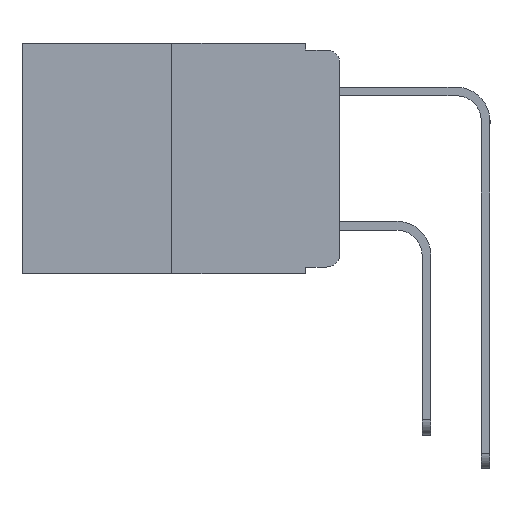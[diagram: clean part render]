
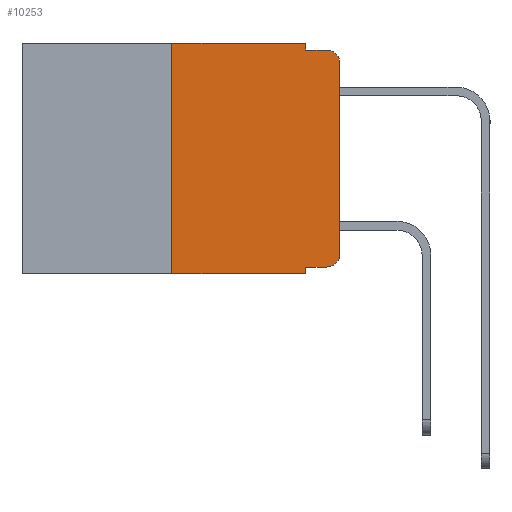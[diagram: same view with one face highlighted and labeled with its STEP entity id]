
A CAD part, left-side view. The second image highlights one B-rep face of the part: STEP entity #10253.
In plain terms, the highlighted planar face has unit normal (-1, 0, 0).
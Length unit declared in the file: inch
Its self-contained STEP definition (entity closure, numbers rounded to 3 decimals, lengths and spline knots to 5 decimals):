
#433 = CARTESIAN_POINT ( 'NONE',  ( 0., 0.02, -0.333 ) ) ;
#445 = VERTEX_POINT ( 'NONE', #18085 ) ;
#580 = VERTEX_POINT ( 'NONE', #11649 ) ;
#605 = CARTESIAN_POINT ( 'NONE',  ( 0., 0.051, -0.01 ) ) ;
#754 = ORIENTED_EDGE ( 'NONE', *, *, #6500, .T. ) ;
#1290 = CARTESIAN_POINT ( 'NONE',  ( 0., 0.051, 0. ) ) ;
#1315 = EDGE_CURVE ( 'NONE', #15771, #9281, #1794, .T. ) ;
#1666 = CARTESIAN_POINT ( 'NONE',  ( 0., 0.473, 0. ) ) ;
#1714 = CARTESIAN_POINT ( 'NONE',  ( 0., 0.02, -0.03 ) ) ;
#1794 = LINE ( 'NONE', #10385, #9416 ) ;
#2093 = VECTOR ( 'NONE', #3035, 39.37008 ) ;
#2310 = ORIENTED_EDGE ( 'NONE', *, *, #16106, .F. ) ;
#2393 = CARTESIAN_POINT ( 'NONE',  ( 0., 0., -0.03 ) ) ;
#2771 = LINE ( 'NONE', #4228, #17580 ) ;
#2991 = DIRECTION ( 'NONE',  ( -1., 0., 0. ) ) ;
#3035 = DIRECTION ( 'NONE',  ( 0., -1., 0. ) ) ;
#3064 = EDGE_CURVE ( 'NONE', #445, #11190, #14679, .T. ) ;
#3066 = ORIENTED_EDGE ( 'NONE', *, *, #5464, .T. ) ;
#3244 = DIRECTION ( 'NONE',  ( 1., 0., 0. ) ) ;
#3263 = CARTESIAN_POINT ( 'NONE',  ( 0., 0., 0. ) ) ;
#3291 = DIRECTION ( 'NONE',  ( 0., 0., -1. ) ) ;
#4115 = EDGE_CURVE ( 'NONE', #5108, #580, #12930, .T. ) ;
#4228 = CARTESIAN_POINT ( 'NONE',  ( 0., 0.25, 0. ) ) ;
#4247 = AXIS2_PLACEMENT_3D ( 'NONE', #1714, #12089, #3291 ) ;
#4293 = EDGE_CURVE ( 'NONE', #14950, #5108, #17659, .T. ) ;
#4576 = CARTESIAN_POINT ( 'NONE',  ( 0., 0.473, 0. ) ) ;
#4803 = DIRECTION ( 'NONE',  ( 0., 0., 1. ) ) ;
#4983 = DIRECTION ( 'NONE',  ( 0., -1., 0. ) ) ;
#5108 = VERTEX_POINT ( 'NONE', #433 ) ;
#5315 = EDGE_CURVE ( 'NONE', #14950, #11190, #12246, .T. ) ;
#5464 = EDGE_CURVE ( 'NONE', #6756, #9281, #12873, .T. ) ;
#5842 = VECTOR ( 'NONE', #6880, 39.37008 ) ;
#5884 = ORIENTED_EDGE ( 'NONE', *, *, #4293, .T. ) ;
#6154 = LINE ( 'NONE', #4576, #2093 ) ;
#6315 = LINE ( 'NONE', #8388, #5842 ) ;
#6500 = EDGE_CURVE ( 'NONE', #580, #6756, #9173, .T. ) ;
#6756 = VERTEX_POINT ( 'NONE', #2393 ) ;
#6880 = DIRECTION ( 'NONE',  ( 0., 0., -1. ) ) ;
#7239 = DIRECTION ( 'NONE',  ( 0., -1., 0. ) ) ;
#7296 = DIRECTION ( 'NONE',  ( 0., 0., 1. ) ) ;
#7792 = AXIS2_PLACEMENT_3D ( 'NONE', #11841, #2991, #13220 ) ;
#7902 = CARTESIAN_POINT ( 'NONE',  ( 0., 0.051, -0.333 ) ) ;
#8388 = CARTESIAN_POINT ( 'NONE',  ( 0., 0.051, 0. ) ) ;
#8506 = VECTOR ( 'NONE', #14509, 39.37008 ) ;
#8715 = VECTOR ( 'NONE', #4803, 39.37008 ) ;
#9173 = LINE ( 'NONE', #3263, #8715 ) ;
#9281 = VERTEX_POINT ( 'NONE', #16473 ) ;
#9350 = DIRECTION ( 'NONE',  ( 0., -1., 0. ) ) ;
#9416 = VECTOR ( 'NONE', #7239, 39.37008 ) ;
#9873 = ORIENTED_EDGE ( 'NONE', *, *, #11886, .F. ) ;
#10145 = ORIENTED_EDGE ( 'NONE', *, *, #12331, .F. ) ;
#10253 = ADVANCED_FACE ( 'NONE', ( #17227 ), #10686, .F. ) ;
#10344 = ORIENTED_EDGE ( 'NONE', *, *, #4115, .T. ) ;
#10385 = CARTESIAN_POINT ( 'NONE',  ( 0., 0.051, -0.01 ) ) ;
#10607 = VECTOR ( 'NONE', #4983, 39.37008 ) ;
#10686 = PLANE ( 'NONE',  #14241 ) ;
#10785 = VECTOR ( 'NONE', #9350, 39.37008 ) ;
#10928 = CARTESIAN_POINT ( 'NONE',  ( 0., 0.473, -0.343 ) ) ;
#11190 = VERTEX_POINT ( 'NONE', #16970 ) ;
#11649 = CARTESIAN_POINT ( 'NONE',  ( 0., 0., -0.313 ) ) ;
#11841 = CARTESIAN_POINT ( 'NONE',  ( 0., 0.02, -0.313 ) ) ;
#11859 = VERTEX_POINT ( 'NONE', #18427 ) ;
#11886 = EDGE_CURVE ( 'NONE', #445, #13975, #2771, .T. ) ;
#12089 = DIRECTION ( 'NONE',  ( -1., 0., 0. ) ) ;
#12246 = LINE ( 'NONE', #1290, #8506 ) ;
#12331 = EDGE_CURVE ( 'NONE', #11859, #15771, #6315, .T. ) ;
#12773 = CARTESIAN_POINT ( 'NONE',  ( 0., 0.25, 0. ) ) ;
#12873 = CIRCLE ( 'NONE', #4247, 0.02 ) ;
#12930 = CIRCLE ( 'NONE', #7792, 0.02 ) ;
#13220 = DIRECTION ( 'NONE',  ( 0., 0., -1. ) ) ;
#13321 = ORIENTED_EDGE ( 'NONE', *, *, #5315, .F. ) ;
#13367 = EDGE_LOOP ( 'NONE', ( #754, #3066, #15690, #10145, #2310, #9873, #13530, #13321, #5884, #10344 ) ) ;
#13455 = DIRECTION ( 'NONE',  ( 0., 0., -1. ) ) ;
#13530 = ORIENTED_EDGE ( 'NONE', *, *, #3064, .T. ) ;
#13975 = VERTEX_POINT ( 'NONE', #12773 ) ;
#14241 = AXIS2_PLACEMENT_3D ( 'NONE', #1666, #3244, #13455 ) ;
#14509 = DIRECTION ( 'NONE',  ( 0., 0., -1. ) ) ;
#14664 = CARTESIAN_POINT ( 'NONE',  ( 0., 0.051, -0.333 ) ) ;
#14679 = LINE ( 'NONE', #10928, #10607 ) ;
#14950 = VERTEX_POINT ( 'NONE', #14664 ) ;
#15690 = ORIENTED_EDGE ( 'NONE', *, *, #1315, .F. ) ;
#15771 = VERTEX_POINT ( 'NONE', #605 ) ;
#16106 = EDGE_CURVE ( 'NONE', #13975, #11859, #6154, .T. ) ;
#16473 = CARTESIAN_POINT ( 'NONE',  ( 0., 0.02, -0.01 ) ) ;
#16970 = CARTESIAN_POINT ( 'NONE',  ( 0., 0.051, -0.343 ) ) ;
#17227 = FACE_OUTER_BOUND ( 'NONE', #13367, .T. ) ;
#17580 = VECTOR ( 'NONE', #7296, 39.37008 ) ;
#17659 = LINE ( 'NONE', #7902, #10785 ) ;
#18085 = CARTESIAN_POINT ( 'NONE',  ( 0., 0.25, -0.343 ) ) ;
#18427 = CARTESIAN_POINT ( 'NONE',  ( 0., 0.051, 0. ) ) ;
